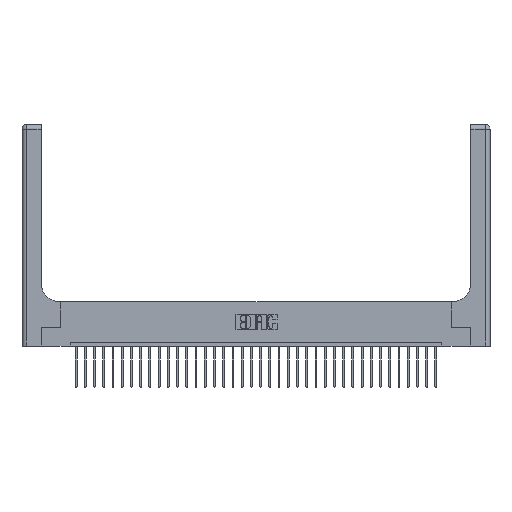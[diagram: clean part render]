
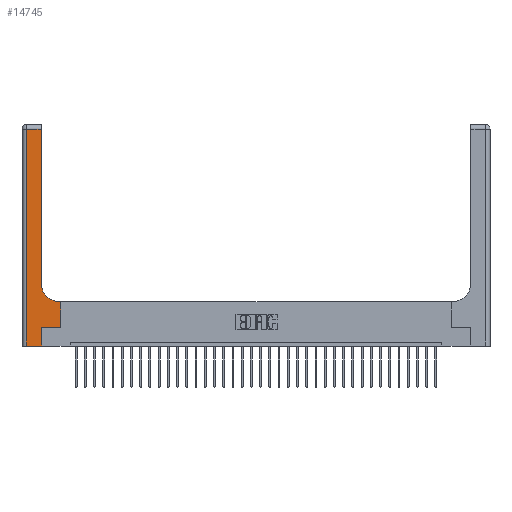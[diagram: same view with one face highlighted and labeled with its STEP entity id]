
A CAD part, top view. The second image highlights one B-rep face of the part: STEP entity #14745.
In plain terms, the highlighted planar face has unit normal (0, 0, 1).
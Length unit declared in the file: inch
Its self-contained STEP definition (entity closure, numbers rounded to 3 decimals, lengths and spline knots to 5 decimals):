
#470 = CARTESIAN_POINT ( 'NONE',  ( 0.265, 0.25, 0.37 ) ) ;
#558 = VECTOR ( 'NONE', #7251, 39.37008 ) ;
#738 = CARTESIAN_POINT ( 'NONE',  ( 0.528, 0.25, 0.37 ) ) ;
#925 = VERTEX_POINT ( 'NONE', #23329 ) ;
#1063 = VERTEX_POINT ( 'NONE', #470 ) ;
#1117 = DIRECTION ( 'NONE',  ( 0., -1., 0. ) ) ;
#1232 = VECTOR ( 'NONE', #1117, 39.37008 ) ;
#1363 = LINE ( 'NONE', #27280, #8343 ) ;
#1484 = EDGE_CURVE ( 'NONE', #14654, #925, #15995, .T. ) ;
#2962 = DIRECTION ( 'NONE',  ( -1., 0., 0. ) ) ;
#3512 = VECTOR ( 'NONE', #19549, 39.37008 ) ;
#3791 = CARTESIAN_POINT ( 'NONE',  ( 0.26, 0.6, 0.37 ) ) ;
#4003 = DIRECTION ( 'NONE',  ( -1., 0., 0. ) ) ;
#4024 = CARTESIAN_POINT ( 'NONE',  ( 0.26, 3., 0.37 ) ) ;
#4168 = ORIENTED_EDGE ( 'NONE', *, *, #15579, .T. ) ;
#4305 = VERTEX_POINT ( 'NONE', #18565 ) ;
#4440 = ORIENTED_EDGE ( 'NONE', *, *, #19949, .T. ) ;
#5631 = VECTOR ( 'NONE', #29485, 39.37008 ) ;
#6601 = CARTESIAN_POINT ( 'NONE',  ( 0.51, 0.85, 0.37 ) ) ;
#7251 = DIRECTION ( 'NONE',  ( 0., 1., 0. ) ) ;
#7408 = CARTESIAN_POINT ( 'NONE',  ( 0.51, 0.6, 0.37 ) ) ;
#8227 = FACE_OUTER_BOUND ( 'NONE', #21884, .T. ) ;
#8343 = VECTOR ( 'NONE', #20300, 39.37008 ) ;
#8680 = ORIENTED_EDGE ( 'NONE', *, *, #28408, .T. ) ;
#9915 = CARTESIAN_POINT ( 'NONE',  ( 0.265, 0., 0.37 ) ) ;
#9924 = CARTESIAN_POINT ( 'NONE',  ( 0.26, 2.94, 0.37 ) ) ;
#11277 = DIRECTION ( 'NONE',  ( 0., 1., 0. ) ) ;
#11414 = ORIENTED_EDGE ( 'NONE', *, *, #27372, .T. ) ;
#12190 = PLANE ( 'NONE',  #15268 ) ;
#13020 = EDGE_CURVE ( 'NONE', #1063, #14654, #1363, .T. ) ;
#13873 = CARTESIAN_POINT ( 'NONE',  ( 0.265, 0., 0.37 ) ) ;
#14186 = VERTEX_POINT ( 'NONE', #9924 ) ;
#14536 = EDGE_CURVE ( 'NONE', #23891, #1063, #19203, .T. ) ;
#14654 = VERTEX_POINT ( 'NONE', #738 ) ;
#14745 = ADVANCED_FACE ( 'NONE', ( #8227 ), #12190, .F. ) ;
#15268 = AXIS2_PLACEMENT_3D ( 'NONE', #16998, #26548, #2962 ) ;
#15341 = ORIENTED_EDGE ( 'NONE', *, *, #13020, .T. ) ;
#15579 = EDGE_CURVE ( 'NONE', #24153, #14186, #26463, .T. ) ;
#15995 = LINE ( 'NONE', #30255, #20693 ) ;
#16190 = ORIENTED_EDGE ( 'NONE', *, *, #19092, .T. ) ;
#16283 = LINE ( 'NONE', #29624, #27600 ) ;
#16998 = CARTESIAN_POINT ( 'NONE',  ( 0., 3., 0.37 ) ) ;
#17050 = AXIS2_PLACEMENT_3D ( 'NONE', #6601, #29884, #29687 ) ;
#17062 = CARTESIAN_POINT ( 'NONE',  ( 0., 0., 0.37 ) ) ;
#18565 = CARTESIAN_POINT ( 'NONE',  ( 0.06, 0., 0.37 ) ) ;
#19092 = EDGE_CURVE ( 'NONE', #20206, #24153, #19666, .T. ) ;
#19203 = LINE ( 'NONE', #13873, #558 ) ;
#19549 = DIRECTION ( 'NONE',  ( 1., 0., 0. ) ) ;
#19589 = CARTESIAN_POINT ( 'NONE',  ( 0.06, 3., 0.37 ) ) ;
#19666 = CIRCLE ( 'NONE', #17050, 0.25 ) ;
#19949 = EDGE_CURVE ( 'NONE', #4305, #23891, #23951, .T. ) ;
#20206 = VERTEX_POINT ( 'NONE', #7408 ) ;
#20300 = DIRECTION ( 'NONE',  ( 1., 0., 0. ) ) ;
#20525 = VECTOR ( 'NONE', #4003, 39.37008 ) ;
#20598 = EDGE_CURVE ( 'NONE', #14186, #22270, #16283, .T. ) ;
#20693 = VECTOR ( 'NONE', #11277, 39.37008 ) ;
#21419 = ORIENTED_EDGE ( 'NONE', *, *, #20598, .T. ) ;
#21884 = EDGE_LOOP ( 'NONE', ( #4168, #21419, #11414, #4440, #22295, #15341, #24540, #8680, #16190 ) ) ;
#22270 = VERTEX_POINT ( 'NONE', #29934 ) ;
#22295 = ORIENTED_EDGE ( 'NONE', *, *, #14536, .T. ) ;
#22316 = DIRECTION ( 'NONE',  ( -1., 0., 0. ) ) ;
#23329 = CARTESIAN_POINT ( 'NONE',  ( 0.528, 0.6, 0.37 ) ) ;
#23891 = VERTEX_POINT ( 'NONE', #9915 ) ;
#23951 = LINE ( 'NONE', #17062, #3512 ) ;
#24153 = VERTEX_POINT ( 'NONE', #26820 ) ;
#24540 = ORIENTED_EDGE ( 'NONE', *, *, #1484, .T. ) ;
#26463 = LINE ( 'NONE', #4024, #5631 ) ;
#26548 = DIRECTION ( 'NONE',  ( 0., 0., -1. ) ) ;
#26820 = CARTESIAN_POINT ( 'NONE',  ( 0.26, 0.85, 0.37 ) ) ;
#27280 = CARTESIAN_POINT ( 'NONE',  ( 0.265, 0.25, 0.37 ) ) ;
#27372 = EDGE_CURVE ( 'NONE', #22270, #4305, #29777, .T. ) ;
#27516 = LINE ( 'NONE', #3791, #20525 ) ;
#27600 = VECTOR ( 'NONE', #22316, 39.37008 ) ;
#28408 = EDGE_CURVE ( 'NONE', #925, #20206, #27516, .T. ) ;
#29485 = DIRECTION ( 'NONE',  ( 0., 1., 0. ) ) ;
#29624 = CARTESIAN_POINT ( 'NONE',  ( 0., 2.94, 0.37 ) ) ;
#29687 = DIRECTION ( 'NONE',  ( 1., 0., 0. ) ) ;
#29777 = LINE ( 'NONE', #19589, #1232 ) ;
#29884 = DIRECTION ( 'NONE',  ( 0., 0., -1. ) ) ;
#29934 = CARTESIAN_POINT ( 'NONE',  ( 0.06, 2.94, 0.37 ) ) ;
#30255 = CARTESIAN_POINT ( 'NONE',  ( 0.528, 0.25, 0.37 ) ) ;
